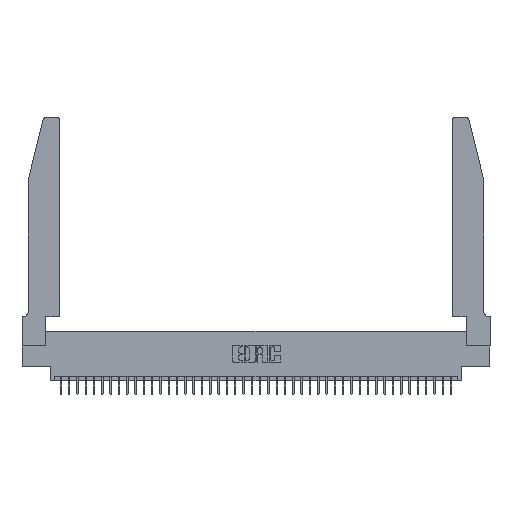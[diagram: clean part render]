
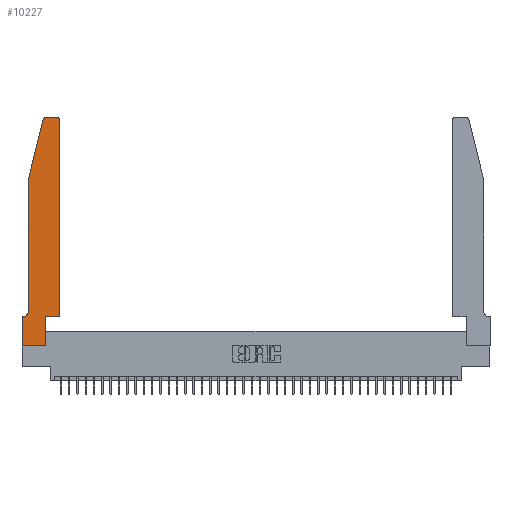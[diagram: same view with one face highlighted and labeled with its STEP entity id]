
A CAD part, top view. The second image highlights one B-rep face of the part: STEP entity #10227.
In plain terms, the highlighted planar face has unit normal (0, 0, 1).
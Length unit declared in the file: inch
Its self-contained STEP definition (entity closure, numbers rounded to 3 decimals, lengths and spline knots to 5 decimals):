
#1312 = DIRECTION ( 'NONE',  ( 0., 0., 1. ) ) ;
#1627 = CARTESIAN_POINT ( 'NONE',  ( 0.4505, 0.35, 0.37 ) ) ;
#2050 = VECTOR ( 'NONE', #29710, 39.37008 ) ;
#2801 = CIRCLE ( 'NONE', #41558, 0.03 ) ;
#3219 = DIRECTION ( 'NONE',  ( 0., 1., 0. ) ) ;
#3470 = ORIENTED_EDGE ( 'NONE', *, *, #31512, .T. ) ;
#3507 = ORIENTED_EDGE ( 'NONE', *, *, #15318, .T. ) ;
#3794 = CARTESIAN_POINT ( 'NONE',  ( 0.2865, 0., 0.37 ) ) ;
#4121 = LINE ( 'NONE', #30373, #19267 ) ;
#4151 = CARTESIAN_POINT ( 'NONE',  ( 0.284, 2.72, 0.37 ) ) ;
#4203 = CIRCLE ( 'NONE', #21097, 0.07 ) ;
#4497 = VERTEX_POINT ( 'NONE', #29936 ) ;
#4500 = CIRCLE ( 'NONE', #30468, 0.03 ) ;
#5015 = EDGE_CURVE ( 'NONE', #33193, #4497, #24992, .T. ) ;
#5032 = LINE ( 'NONE', #21665, #38379 ) ;
#5701 = ORIENTED_EDGE ( 'NONE', *, *, #15819, .T. ) ;
#6049 = VERTEX_POINT ( 'NONE', #18365 ) ;
#6460 = CARTESIAN_POINT ( 'NONE',  ( 0.2865, 0.35, 0.37 ) ) ;
#6463 = EDGE_CURVE ( 'NONE', #13091, #36675, #4203, .T. ) ;
#6800 = VECTOR ( 'NONE', #17427, 39.37008 ) ;
#7385 = DIRECTION ( 'NONE',  ( 1., 0., 0. ) ) ;
#7754 = DIRECTION ( 'NONE',  ( -1., 0., 0. ) ) ;
#7803 = LINE ( 'NONE', #40068, #6800 ) ;
#7869 = LINE ( 'NONE', #33879, #31663 ) ;
#8042 = VECTOR ( 'NONE', #14804, 39.37008 ) ;
#8769 = DIRECTION ( 'NONE',  ( 0., 1., 0. ) ) ;
#9350 = ORIENTED_EDGE ( 'NONE', *, *, #21414, .T. ) ;
#9362 = CARTESIAN_POINT ( 'NONE',  ( 0.0755, 2., 0.37 ) ) ;
#9903 = VERTEX_POINT ( 'NONE', #41379 ) ;
#10227 = ADVANCED_FACE ( 'NONE', ( #34218 ), #33119, .T. ) ;
#10829 = DIRECTION ( 'NONE',  ( 0., 0., -1. ) ) ;
#11193 = ORIENTED_EDGE ( 'NONE', *, *, #6463, .T. ) ;
#11206 = DIRECTION ( 'NONE',  ( 1., 0., 0. ) ) ;
#11586 = LINE ( 'NONE', #26480, #2050 ) ;
#12177 = EDGE_CURVE ( 'NONE', #32713, #23494, #4500, .T. ) ;
#12756 = LINE ( 'NONE', #1627, #37556 ) ;
#13091 = VERTEX_POINT ( 'NONE', #16182 ) ;
#13670 = CARTESIAN_POINT ( 'NONE',  ( 0., 0.35, 0.37 ) ) ;
#14531 = DIRECTION ( 'NONE',  ( 1., 0., 0. ) ) ;
#14804 = DIRECTION ( 'NONE',  ( -1., 0., 0. ) ) ;
#15318 = EDGE_CURVE ( 'NONE', #37909, #19943, #7803, .T. ) ;
#15819 = EDGE_CURVE ( 'NONE', #19943, #13091, #37571, .T. ) ;
#16182 = CARTESIAN_POINT ( 'NONE',  ( 0.0755, 0.42, 0.37 ) ) ;
#16444 = ORIENTED_EDGE ( 'NONE', *, *, #32072, .T. ) ;
#16662 = ORIENTED_EDGE ( 'NONE', *, *, #21488, .T. ) ;
#17427 = DIRECTION ( 'NONE',  ( -0.239, -0.971, 0. ) ) ;
#18090 = CARTESIAN_POINT ( 'NONE',  ( 0.0755, 0.35, 0.37 ) ) ;
#18145 = VERTEX_POINT ( 'NONE', #37313 ) ;
#18165 = CARTESIAN_POINT ( 'NONE',  ( 0.4205, 2.75, 0.37 ) ) ;
#18308 = ORIENTED_EDGE ( 'NONE', *, *, #12177, .T. ) ;
#18365 = CARTESIAN_POINT ( 'NONE',  ( 0.284, 2.75, 0.37 ) ) ;
#19267 = VECTOR ( 'NONE', #7754, 39.37008 ) ;
#19451 = EDGE_CURVE ( 'NONE', #4497, #9903, #12756, .T. ) ;
#19943 = VERTEX_POINT ( 'NONE', #30650 ) ;
#20184 = CARTESIAN_POINT ( 'NONE',  ( 0.4505, 2.72, 0.37 ) ) ;
#20209 = DIRECTION ( 'NONE',  ( 1., 0., 0. ) ) ;
#20618 = CARTESIAN_POINT ( 'NONE',  ( 0.4205, 2.72, 0.37 ) ) ;
#20726 = CARTESIAN_POINT ( 'NONE',  ( 0., 0.35, 0.37 ) ) ;
#21097 = AXIS2_PLACEMENT_3D ( 'NONE', #30224, #10829, #33516 ) ;
#21142 = EDGE_CURVE ( 'NONE', #35537, #18145, #11586, .T. ) ;
#21414 = EDGE_CURVE ( 'NONE', #36675, #35537, #33868, .T. ) ;
#21488 = EDGE_CURVE ( 'NONE', #9903, #32713, #5032, .T. ) ;
#21665 = CARTESIAN_POINT ( 'NONE',  ( 0.4505, 0.35, 0.37 ) ) ;
#22460 = ORIENTED_EDGE ( 'NONE', *, *, #5015, .T. ) ;
#23494 = VERTEX_POINT ( 'NONE', #18165 ) ;
#23911 = DIRECTION ( 'NONE',  ( 1., 0., 0. ) ) ;
#24992 = LINE ( 'NONE', #6460, #41163 ) ;
#25476 = ORIENTED_EDGE ( 'NONE', *, *, #21142, .T. ) ;
#26080 = EDGE_CURVE ( 'NONE', #23494, #6049, #4121, .T. ) ;
#26480 = CARTESIAN_POINT ( 'NONE',  ( 0., 0., 0.37 ) ) ;
#26751 = DIRECTION ( 'NONE',  ( 0., 0., 1. ) ) ;
#27993 = VECTOR ( 'NONE', #41740, 39.37008 ) ;
#29710 = DIRECTION ( 'NONE',  ( 0., -1., 0. ) ) ;
#29936 = CARTESIAN_POINT ( 'NONE',  ( 0.2865, 0.35, 0.37 ) ) ;
#30154 = AXIS2_PLACEMENT_3D ( 'NONE', #13670, #39577, #20209 ) ;
#30224 = CARTESIAN_POINT ( 'NONE',  ( 0.0055, 0.42, 0.37 ) ) ;
#30373 = CARTESIAN_POINT ( 'NONE',  ( 0.2605, 2.75, 0.37 ) ) ;
#30468 = AXIS2_PLACEMENT_3D ( 'NONE', #20618, #1312, #23911 ) ;
#30650 = CARTESIAN_POINT ( 'NONE',  ( 0.0755, 2., 0.37 ) ) ;
#31512 = EDGE_CURVE ( 'NONE', #18145, #33193, #7869, .T. ) ;
#31663 = VECTOR ( 'NONE', #11206, 39.37008 ) ;
#32072 = EDGE_CURVE ( 'NONE', #6049, #37909, #2801, .T. ) ;
#32713 = VERTEX_POINT ( 'NONE', #20184 ) ;
#33119 = PLANE ( 'NONE',  #30154 ) ;
#33193 = VERTEX_POINT ( 'NONE', #3794 ) ;
#33516 = DIRECTION ( 'NONE',  ( -1., 0., 0. ) ) ;
#33868 = LINE ( 'NONE', #18090, #8042 ) ;
#33879 = CARTESIAN_POINT ( 'NONE',  ( 0., 0., 0.37 ) ) ;
#34218 = FACE_OUTER_BOUND ( 'NONE', #34563, .T. ) ;
#34563 = EDGE_LOOP ( 'NONE', ( #35662, #16444, #3507, #5701, #11193, #9350, #25476, #3470, #22460, #39689, #16662, #18308 ) ) ;
#35537 = VERTEX_POINT ( 'NONE', #20726 ) ;
#35662 = ORIENTED_EDGE ( 'NONE', *, *, #26080, .T. ) ;
#36675 = VERTEX_POINT ( 'NONE', #38736 ) ;
#36880 = CARTESIAN_POINT ( 'NONE',  ( 0.25487, 2.72718, 0.37 ) ) ;
#37313 = CARTESIAN_POINT ( 'NONE',  ( 0., 0., 0.37 ) ) ;
#37556 = VECTOR ( 'NONE', #14531, 39.37008 ) ;
#37571 = LINE ( 'NONE', #9362, #27993 ) ;
#37909 = VERTEX_POINT ( 'NONE', #36880 ) ;
#38379 = VECTOR ( 'NONE', #8769, 39.37008 ) ;
#38736 = CARTESIAN_POINT ( 'NONE',  ( 0.0055, 0.35, 0.37 ) ) ;
#39577 = DIRECTION ( 'NONE',  ( 0., 0., 1. ) ) ;
#39689 = ORIENTED_EDGE ( 'NONE', *, *, #19451, .T. ) ;
#40068 = CARTESIAN_POINT ( 'NONE',  ( 0.0755, 2., 0.37 ) ) ;
#41163 = VECTOR ( 'NONE', #3219, 39.37008 ) ;
#41379 = CARTESIAN_POINT ( 'NONE',  ( 0.4505, 0.35, 0.37 ) ) ;
#41558 = AXIS2_PLACEMENT_3D ( 'NONE', #4151, #26751, #7385 ) ;
#41740 = DIRECTION ( 'NONE',  ( 0., -1., 0. ) ) ;
